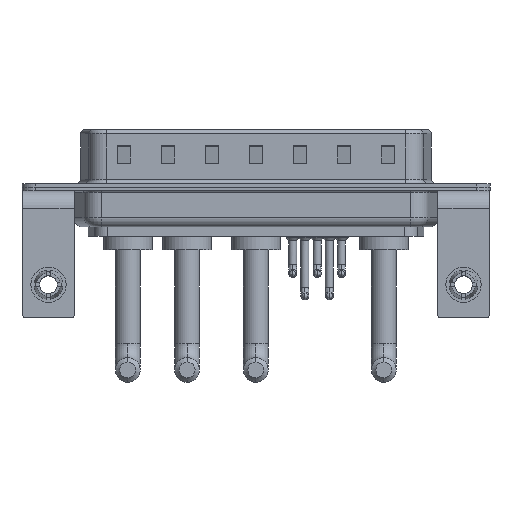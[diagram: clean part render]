
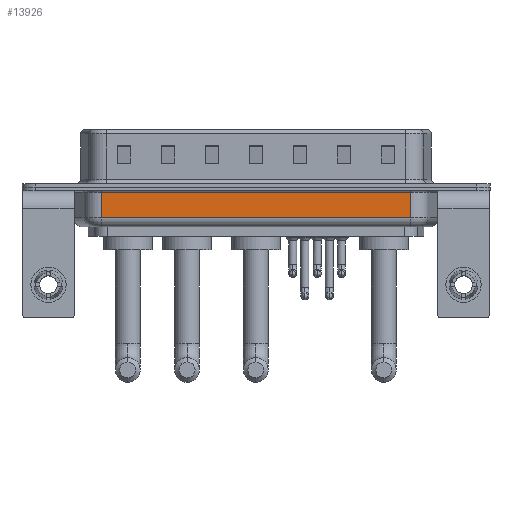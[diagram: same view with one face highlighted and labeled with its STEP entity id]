
A CAD part, front view. The second image highlights one B-rep face of the part: STEP entity #13926.
In plain terms, the highlighted planar face has unit normal (0, -1, 0).
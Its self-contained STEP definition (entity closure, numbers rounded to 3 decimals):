
#209 = VERTEX_POINT ( 'NONE', #21950 ) ;
#403 = DIRECTION ( 'NONE',  ( 0., 1., 0. ) ) ;
#1360 = CARTESIAN_POINT ( 'NONE',  ( 6.006, -5.35, -3.5 ) ) ;
#1500 = CARTESIAN_POINT ( 'NONE',  ( 6.006, -5.35, -4.5 ) ) ;
#3202 = CARTESIAN_POINT ( 'NONE',  ( 41.044, -5.35, -4.5 ) ) ;
#3557 = DIRECTION ( 'NONE',  ( 0., 0., 1. ) ) ;
#5735 = CARTESIAN_POINT ( 'NONE',  ( 41.044, -5.35, -3.5 ) ) ;
#7166 = VECTOR ( 'NONE', #18552, 1000. ) ;
#7581 = LINE ( 'NONE', #1360, #18617 ) ;
#7650 = CARTESIAN_POINT ( 'NONE',  ( 6.006, -5.35, -4.5 ) ) ;
#8966 = EDGE_CURVE ( 'NONE', #209, #13460, #22765, .T. ) ;
#9096 = DIRECTION ( 'NONE',  ( 1., 0., 0. ) ) ;
#9325 = EDGE_CURVE ( 'NONE', #10001, #13460, #12872, .T. ) ;
#9584 = VECTOR ( 'NONE', #3557, 1000. ) ;
#9794 = FACE_OUTER_BOUND ( 'NONE', #19568, .T. ) ;
#9964 = VERTEX_POINT ( 'NONE', #5735 ) ;
#9994 = ORIENTED_EDGE ( 'NONE', *, *, #20228, .T. ) ;
#10001 = VERTEX_POINT ( 'NONE', #15451 ) ;
#10539 = LINE ( 'NONE', #3202, #18433 ) ;
#11746 = EDGE_CURVE ( 'NONE', #209, #9964, #7581, .T. ) ;
#12872 = LINE ( 'NONE', #14629, #7166 ) ;
#13460 = VERTEX_POINT ( 'NONE', #22848 ) ;
#13712 = PLANE ( 'NONE',  #21886 ) ;
#13926 = ADVANCED_FACE ( 'NONE', ( #9794 ), #13712, .F. ) ;
#14629 = CARTESIAN_POINT ( 'NONE',  ( 6.006, -5.35, -0.65 ) ) ;
#15451 = CARTESIAN_POINT ( 'NONE',  ( 41.044, -5.35, -0.65 ) ) ;
#16712 = ORIENTED_EDGE ( 'NONE', *, *, #11746, .T. ) ;
#18433 = VECTOR ( 'NONE', #23816, 1000. ) ;
#18552 = DIRECTION ( 'NONE',  ( -1., 0., 0. ) ) ;
#18617 = VECTOR ( 'NONE', #9096, 1000. ) ;
#19568 = EDGE_LOOP ( 'NONE', ( #20944, #16712, #9994, #23448 ) ) ;
#20228 = EDGE_CURVE ( 'NONE', #9964, #10001, #10539, .T. ) ;
#20944 = ORIENTED_EDGE ( 'NONE', *, *, #8966, .F. ) ;
#21886 = AXIS2_PLACEMENT_3D ( 'NONE', #7650, #403, #23439 ) ;
#21950 = CARTESIAN_POINT ( 'NONE',  ( 6.006, -5.35, -3.5 ) ) ;
#22765 = LINE ( 'NONE', #1500, #9584 ) ;
#22848 = CARTESIAN_POINT ( 'NONE',  ( 6.006, -5.35, -0.65 ) ) ;
#23439 = DIRECTION ( 'NONE',  ( 0., 0., 1. ) ) ;
#23448 = ORIENTED_EDGE ( 'NONE', *, *, #9325, .T. ) ;
#23816 = DIRECTION ( 'NONE',  ( 0., 0., 1. ) ) ;
